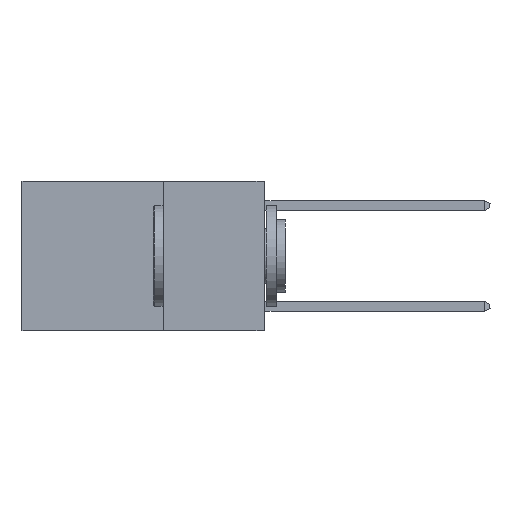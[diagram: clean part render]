
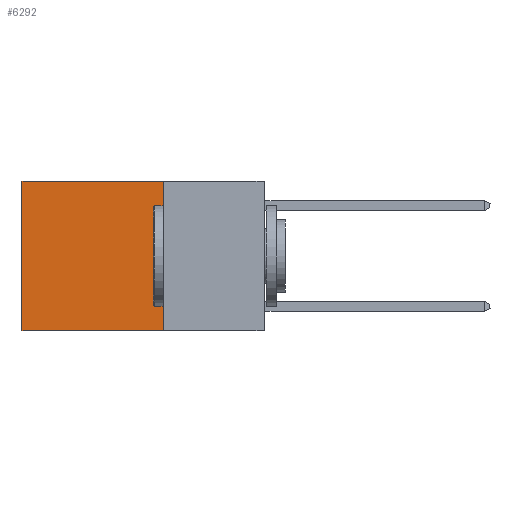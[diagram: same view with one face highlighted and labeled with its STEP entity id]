
A CAD part, left-side view. The second image highlights one B-rep face of the part: STEP entity #6292.
In plain terms, the highlighted planar face has unit normal (-1, 0, 0).
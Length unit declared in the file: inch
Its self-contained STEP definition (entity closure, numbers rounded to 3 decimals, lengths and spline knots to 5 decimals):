
#228 = VERTEX_POINT ( 'NONE', #1953 ) ;
#798 = DIRECTION ( 'NONE',  ( 0., 1., 0. ) ) ;
#1827 = VECTOR ( 'NONE', #10656, 39.37008 ) ;
#1929 = CARTESIAN_POINT ( 'NONE',  ( 0.2625, 0.6, -0.37 ) ) ;
#1953 = CARTESIAN_POINT ( 'NONE',  ( 0.2625, 0.25, 0. ) ) ;
#2350 = EDGE_CURVE ( 'NONE', #6024, #10838, #3083, .T. ) ;
#3083 = LINE ( 'NONE', #3232, #15228 ) ;
#3101 = ORIENTED_EDGE ( 'NONE', *, *, #6443, .F. ) ;
#3232 = CARTESIAN_POINT ( 'NONE',  ( 0.2625, 0.25, -0.37 ) ) ;
#3756 = CARTESIAN_POINT ( 'NONE',  ( 0.2625, 0.6, 0. ) ) ;
#5232 = DIRECTION ( 'NONE',  ( 1., 0., 0. ) ) ;
#5233 = VECTOR ( 'NONE', #6275, 39.37008 ) ;
#6024 = VERTEX_POINT ( 'NONE', #14777 ) ;
#6275 = DIRECTION ( 'NONE',  ( 0., 1., 0. ) ) ;
#6292 = ADVANCED_FACE ( 'NONE', ( #8944 ), #10916, .F. ) ;
#6443 = EDGE_CURVE ( 'NONE', #228, #6024, #12834, .T. ) ;
#7189 = DIRECTION ( 'NONE',  ( 0., 0., -1. ) ) ;
#7259 = CARTESIAN_POINT ( 'NONE',  ( 0.2625, 0.6, 0. ) ) ;
#7386 = EDGE_LOOP ( 'NONE', ( #11293, #14158, #3101, #14659 ) ) ;
#7665 = CARTESIAN_POINT ( 'NONE',  ( 0.2625, 0.25, 0. ) ) ;
#8154 = CARTESIAN_POINT ( 'NONE',  ( 0.2625, 0.25, 0. ) ) ;
#8383 = VERTEX_POINT ( 'NONE', #3756 ) ;
#8888 = CARTESIAN_POINT ( 'NONE',  ( 0.2625, 0.25, 0. ) ) ;
#8944 = FACE_OUTER_BOUND ( 'NONE', #7386, .T. ) ;
#9014 = DIRECTION ( 'NONE',  ( 0., 0., -1. ) ) ;
#9260 = EDGE_CURVE ( 'NONE', #228, #8383, #14617, .T. ) ;
#9552 = LINE ( 'NONE', #7259, #9622 ) ;
#9622 = VECTOR ( 'NONE', #7189, 39.37008 ) ;
#10656 = DIRECTION ( 'NONE',  ( 0., 0., -1. ) ) ;
#10838 = VERTEX_POINT ( 'NONE', #1929 ) ;
#10916 = PLANE ( 'NONE',  #11882 ) ;
#11293 = ORIENTED_EDGE ( 'NONE', *, *, #14377, .T. ) ;
#11882 = AXIS2_PLACEMENT_3D ( 'NONE', #7665, #5232, #9014 ) ;
#12834 = LINE ( 'NONE', #8154, #1827 ) ;
#14158 = ORIENTED_EDGE ( 'NONE', *, *, #2350, .F. ) ;
#14377 = EDGE_CURVE ( 'NONE', #8383, #10838, #9552, .T. ) ;
#14617 = LINE ( 'NONE', #8888, #5233 ) ;
#14659 = ORIENTED_EDGE ( 'NONE', *, *, #9260, .T. ) ;
#14777 = CARTESIAN_POINT ( 'NONE',  ( 0.2625, 0.25, -0.37 ) ) ;
#15228 = VECTOR ( 'NONE', #798, 39.37008 ) ;
